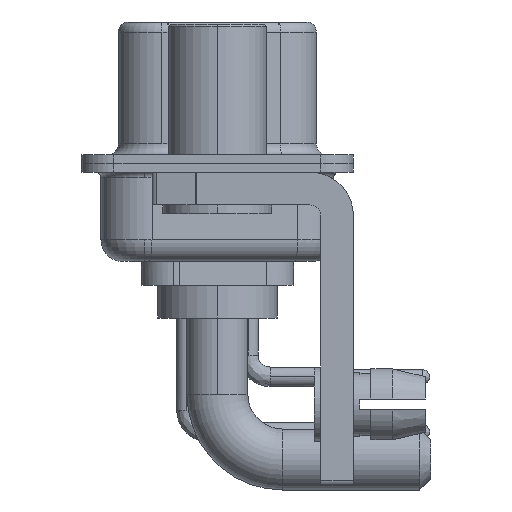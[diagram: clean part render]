
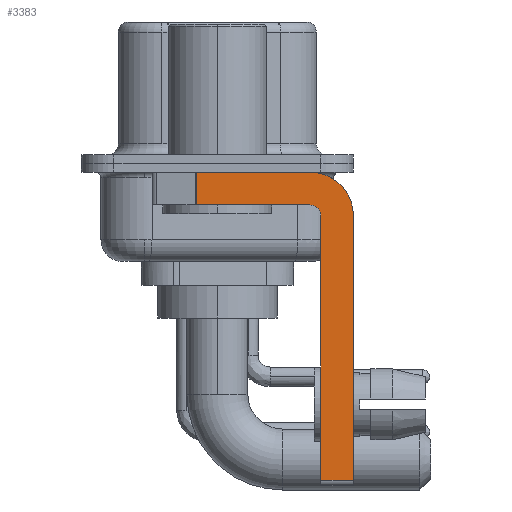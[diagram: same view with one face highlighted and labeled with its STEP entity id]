
A CAD part, left-side view. The second image highlights one B-rep face of the part: STEP entity #3383.
In plain terms, the highlighted planar face has unit normal (-1, 0, 0).
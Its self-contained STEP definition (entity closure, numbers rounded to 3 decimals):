
#214 = DIRECTION ( 'NONE',  ( 0., 0., -1. ) ) ;
#353 = VECTOR ( 'NONE', #27405, 1000. ) ;
#1186 = CIRCLE ( 'NONE', #13873, 0.5 ) ;
#1801 = DIRECTION ( 'NONE',  ( 0., 0., 1. ) ) ;
#1803 = ORIENTED_EDGE ( 'NONE', *, *, #27491, .T. ) ;
#2648 = LINE ( 'NONE', #28257, #27805 ) ;
#2689 = LINE ( 'NONE', #10296, #9644 ) ;
#3383 = ADVANCED_FACE ( 'NONE', ( #25180 ), #15421, .F. ) ;
#3634 = CARTESIAN_POINT ( 'NONE',  ( -2.9, -4.25, -2.4 ) ) ;
#4349 = CARTESIAN_POINT ( 'NONE',  ( -2.9, -4.25, -0.4 ) ) ;
#5267 = ORIENTED_EDGE ( 'NONE', *, *, #13614, .F. ) ;
#5537 = VECTOR ( 'NONE', #20691, 1000. ) ;
#6059 = ORIENTED_EDGE ( 'NONE', *, *, #18136, .F. ) ;
#7354 = CIRCLE ( 'NONE', #24791, 2. ) ;
#7513 = VECTOR ( 'NONE', #31479, 1000. ) ;
#7830 = DIRECTION ( 'NONE',  ( 1., 0., 0. ) ) ;
#8144 = CARTESIAN_POINT ( 'NONE',  ( -2.9, -4.25, -2.4 ) ) ;
#8651 = VERTEX_POINT ( 'NONE', #14185 ) ;
#9317 = CARTESIAN_POINT ( 'NONE',  ( -2.9, -4.25, -2.4 ) ) ;
#9560 = CARTESIAN_POINT ( 'NONE',  ( -2.9, -6.25, -2.4 ) ) ;
#9644 = VECTOR ( 'NONE', #30454, 1000. ) ;
#10296 = CARTESIAN_POINT ( 'NONE',  ( -2.9, 0.978, -1.9 ) ) ;
#10603 = CARTESIAN_POINT ( 'NONE',  ( -2.9, 0.978, -1.9 ) ) ;
#10615 = LINE ( 'NONE', #12767, #5537 ) ;
#10641 = ORIENTED_EDGE ( 'NONE', *, *, #21574, .F. ) ;
#10775 = EDGE_CURVE ( 'NONE', #26606, #20066, #2648, .T. ) ;
#11135 = DIRECTION ( 'NONE',  ( 0., 0., 1. ) ) ;
#11142 = EDGE_CURVE ( 'NONE', #21093, #23549, #25080, .T. ) ;
#12767 = CARTESIAN_POINT ( 'NONE',  ( -2.9, 3., -0.4 ) ) ;
#13614 = EDGE_CURVE ( 'NONE', #18682, #26606, #1186, .T. ) ;
#13873 = AXIS2_PLACEMENT_3D ( 'NONE', #3634, #16852, #1801 ) ;
#14185 = CARTESIAN_POINT ( 'NONE',  ( -2.9, -4.75, -14.55 ) ) ;
#15421 = PLANE ( 'NONE',  #30077 ) ;
#16852 = DIRECTION ( 'NONE',  ( -1., 0., 0. ) ) ;
#18136 = EDGE_CURVE ( 'NONE', #23390, #21093, #7354, .T. ) ;
#18227 = CARTESIAN_POINT ( 'NONE',  ( -2.9, 0.978, -0.4 ) ) ;
#18415 = CARTESIAN_POINT ( 'NONE',  ( -2.9, -4.75, -2.4 ) ) ;
#18682 = VERTEX_POINT ( 'NONE', #18415 ) ;
#19399 = DIRECTION ( 'NONE',  ( 1., 0., 0. ) ) ;
#19490 = ORIENTED_EDGE ( 'NONE', *, *, #10775, .F. ) ;
#19904 = ORIENTED_EDGE ( 'NONE', *, *, #23621, .F. ) ;
#20013 = CARTESIAN_POINT ( 'NONE',  ( -2.9, -4.25, -1.9 ) ) ;
#20066 = VERTEX_POINT ( 'NONE', #10603 ) ;
#20377 = ORIENTED_EDGE ( 'NONE', *, *, #21113, .T. ) ;
#20691 = DIRECTION ( 'NONE',  ( 0., -1., 0. ) ) ;
#20725 = CARTESIAN_POINT ( 'NONE',  ( -2.9, -4.75, -14.8 ) ) ;
#21093 = VERTEX_POINT ( 'NONE', #21417 ) ;
#21113 = EDGE_CURVE ( 'NONE', #8651, #23549, #21249, .T. ) ;
#21249 = LINE ( 'NONE', #31315, #7513 ) ;
#21417 = CARTESIAN_POINT ( 'NONE',  ( -2.9, -6.25, -2.4 ) ) ;
#21574 = EDGE_CURVE ( 'NONE', #8651, #18682, #23856, .T. ) ;
#23146 = DIRECTION ( 'NONE',  ( 0., 1., 0. ) ) ;
#23390 = VERTEX_POINT ( 'NONE', #4349 ) ;
#23549 = VERTEX_POINT ( 'NONE', #30452 ) ;
#23621 = EDGE_CURVE ( 'NONE', #23645, #23390, #10615, .T. ) ;
#23645 = VERTEX_POINT ( 'NONE', #18227 ) ;
#23856 = LINE ( 'NONE', #20725, #28138 ) ;
#24791 = AXIS2_PLACEMENT_3D ( 'NONE', #9317, #19399, #29466 ) ;
#25080 = LINE ( 'NONE', #9560, #353 ) ;
#25180 = FACE_OUTER_BOUND ( 'NONE', #29424, .T. ) ;
#26606 = VERTEX_POINT ( 'NONE', #20013 ) ;
#27405 = DIRECTION ( 'NONE',  ( 0., 0., -1. ) ) ;
#27491 = EDGE_CURVE ( 'NONE', #23645, #20066, #2689, .T. ) ;
#27805 = VECTOR ( 'NONE', #23146, 1000. ) ;
#28138 = VECTOR ( 'NONE', #11135, 1000. ) ;
#28257 = CARTESIAN_POINT ( 'NONE',  ( -2.9, -4.25, -1.9 ) ) ;
#29155 = ORIENTED_EDGE ( 'NONE', *, *, #11142, .F. ) ;
#29424 = EDGE_LOOP ( 'NONE', ( #19904, #1803, #19490, #5267, #10641, #20377, #29155, #6059 ) ) ;
#29466 = DIRECTION ( 'NONE',  ( 0., 0., -1. ) ) ;
#30077 = AXIS2_PLACEMENT_3D ( 'NONE', #8144, #7830, #214 ) ;
#30452 = CARTESIAN_POINT ( 'NONE',  ( -2.9, -6.25, -14.55 ) ) ;
#30454 = DIRECTION ( 'NONE',  ( 0., 0., -1. ) ) ;
#31315 = CARTESIAN_POINT ( 'NONE',  ( -2.9, -4.25, -14.55 ) ) ;
#31479 = DIRECTION ( 'NONE',  ( 0., -1., 0. ) ) ;
